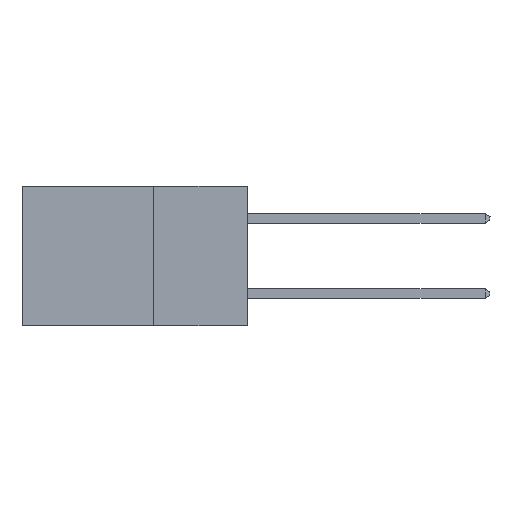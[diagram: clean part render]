
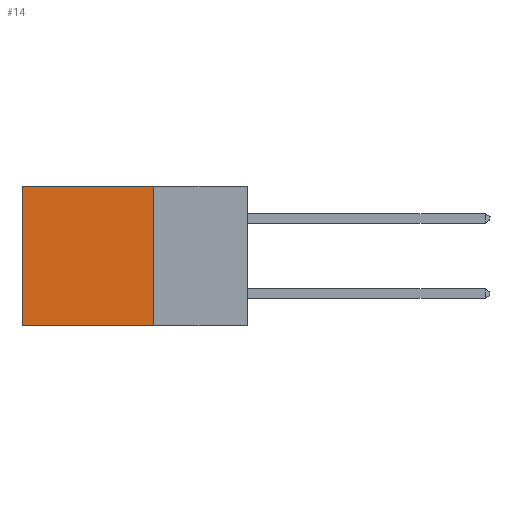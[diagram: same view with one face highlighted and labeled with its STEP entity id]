
A CAD part, left-side view. The second image highlights one B-rep face of the part: STEP entity #14.
In plain terms, the highlighted planar face has unit normal (-1, 0, 0).
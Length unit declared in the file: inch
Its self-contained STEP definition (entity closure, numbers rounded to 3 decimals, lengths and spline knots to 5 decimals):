
#14 = ADVANCED_FACE ( 'NONE', ( #5439 ), #17164, .F. ) ;
#689 = EDGE_CURVE ( 'NONE', #13721, #8769, #8153, .T. ) ;
#1416 = VERTEX_POINT ( 'NONE', #8876 ) ;
#3442 = EDGE_LOOP ( 'NONE', ( #14300, #18881, #11898, #12840 ) ) ;
#3465 = VERTEX_POINT ( 'NONE', #7099 ) ;
#3849 = CARTESIAN_POINT ( 'NONE',  ( 0.2615, 0.25, -0.37 ) ) ;
#4640 = DIRECTION ( 'NONE',  ( 0., 0., -1. ) ) ;
#5439 = FACE_OUTER_BOUND ( 'NONE', #3442, .T. ) ;
#6107 = CARTESIAN_POINT ( 'NONE',  ( 0.2615, 0.25, -0.37 ) ) ;
#6427 = DIRECTION ( 'NONE',  ( 0., 0., -1. ) ) ;
#6880 = CARTESIAN_POINT ( 'NONE',  ( 0.2615, 0.25, 0. ) ) ;
#7099 = CARTESIAN_POINT ( 'NONE',  ( 0.2615, 0.25, -0.37 ) ) ;
#8153 = LINE ( 'NONE', #16776, #17031 ) ;
#8769 = VERTEX_POINT ( 'NONE', #16343 ) ;
#8876 = CARTESIAN_POINT ( 'NONE',  ( 0.2615, 0.6, -0.37 ) ) ;
#8924 = EDGE_CURVE ( 'NONE', #3465, #1416, #18652, .T. ) ;
#9217 = LINE ( 'NONE', #16785, #9579 ) ;
#9579 = VECTOR ( 'NONE', #6427, 39.37008 ) ;
#11271 = DIRECTION ( 'NONE',  ( 0., 1., 0. ) ) ;
#11898 = ORIENTED_EDGE ( 'NONE', *, *, #12370, .F. ) ;
#12370 = EDGE_CURVE ( 'NONE', #13721, #3465, #9217, .T. ) ;
#12752 = LINE ( 'NONE', #18718, #13315 ) ;
#12840 = ORIENTED_EDGE ( 'NONE', *, *, #689, .T. ) ;
#12853 = DIRECTION ( 'NONE',  ( 0., 0., -1. ) ) ;
#13315 = VECTOR ( 'NONE', #12853, 39.37008 ) ;
#13585 = VECTOR ( 'NONE', #11271, 39.37008 ) ;
#13721 = VERTEX_POINT ( 'NONE', #6880 ) ;
#14300 = ORIENTED_EDGE ( 'NONE', *, *, #16524, .T. ) ;
#14926 = DIRECTION ( 'NONE',  ( 1., 0., 0. ) ) ;
#15717 = DIRECTION ( 'NONE',  ( 0., 1., 0. ) ) ;
#16343 = CARTESIAN_POINT ( 'NONE',  ( 0.2615, 0.6, 0. ) ) ;
#16524 = EDGE_CURVE ( 'NONE', #8769, #1416, #12752, .T. ) ;
#16776 = CARTESIAN_POINT ( 'NONE',  ( 0.2615, 0.25, 0. ) ) ;
#16785 = CARTESIAN_POINT ( 'NONE',  ( 0.2615, 0.25, -0.37 ) ) ;
#17031 = VECTOR ( 'NONE', #15717, 39.37008 ) ;
#17164 = PLANE ( 'NONE',  #17931 ) ;
#17931 = AXIS2_PLACEMENT_3D ( 'NONE', #6107, #14926, #4640 ) ;
#18652 = LINE ( 'NONE', #3849, #13585 ) ;
#18718 = CARTESIAN_POINT ( 'NONE',  ( 0.2615, 0.6, -0.37 ) ) ;
#18881 = ORIENTED_EDGE ( 'NONE', *, *, #8924, .F. ) ;
